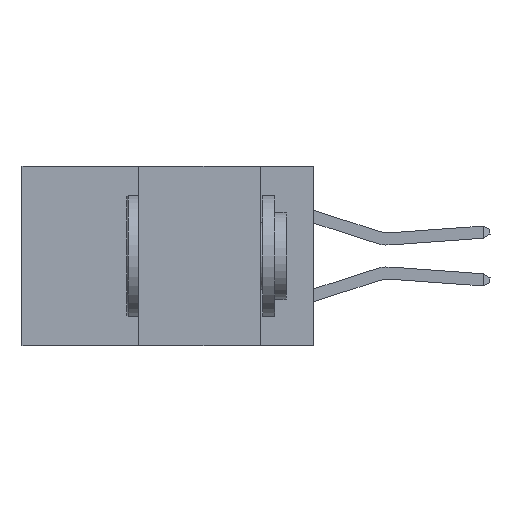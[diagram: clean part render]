
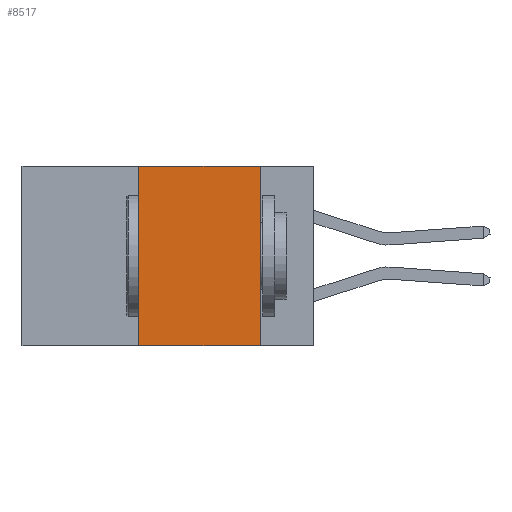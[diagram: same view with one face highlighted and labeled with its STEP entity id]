
A CAD part, left-side view. The second image highlights one B-rep face of the part: STEP entity #8517.
In plain terms, the highlighted planar face has unit normal (-1, 0, 0).
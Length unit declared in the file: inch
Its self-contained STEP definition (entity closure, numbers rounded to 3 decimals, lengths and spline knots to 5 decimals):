
#255 = AXIS2_PLACEMENT_3D ( 'NONE', #11285, #4114, #12508 ) ;
#1003 = LINE ( 'NONE', #3330, #7135 ) ;
#1275 = EDGE_CURVE ( 'NONE', #9500, #12603, #1003, .T. ) ;
#1798 = ORIENTED_EDGE ( 'NONE', *, *, #6247, .T. ) ;
#2509 = DIRECTION ( 'NONE',  ( 0., 0., -1. ) ) ;
#2677 = CARTESIAN_POINT ( 'NONE',  ( 0., 0.11, 0. ) ) ;
#2842 = VECTOR ( 'NONE', #13228, 39.37008 ) ;
#2998 = EDGE_CURVE ( 'NONE', #8325, #4891, #12520, .T. ) ;
#3330 = CARTESIAN_POINT ( 'NONE',  ( 0., 0.36, 0. ) ) ;
#3444 = FACE_OUTER_BOUND ( 'NONE', #7286, .T. ) ;
#3477 = DIRECTION ( 'NONE',  ( 0., 0., 1. ) ) ;
#3578 = CARTESIAN_POINT ( 'NONE',  ( 0., 0.36, -0.37 ) ) ;
#3944 = ORIENTED_EDGE ( 'NONE', *, *, #2998, .F. ) ;
#4114 = DIRECTION ( 'NONE',  ( 1., 0., 0. ) ) ;
#4818 = EDGE_CURVE ( 'NONE', #12603, #8325, #15138, .T. ) ;
#4891 = VERTEX_POINT ( 'NONE', #10911 ) ;
#6031 = LINE ( 'NONE', #7050, #9202 ) ;
#6247 = EDGE_CURVE ( 'NONE', #9500, #4891, #6031, .T. ) ;
#7050 = CARTESIAN_POINT ( 'NONE',  ( 0., 0.6, -0.37 ) ) ;
#7105 = ORIENTED_EDGE ( 'NONE', *, *, #4818, .F. ) ;
#7124 = DIRECTION ( 'NONE',  ( 0., -1., 0. ) ) ;
#7135 = VECTOR ( 'NONE', #3477, 39.37008 ) ;
#7286 = EDGE_LOOP ( 'NONE', ( #3944, #7105, #11058, #1798 ) ) ;
#7630 = PLANE ( 'NONE',  #255 ) ;
#8325 = VERTEX_POINT ( 'NONE', #9747 ) ;
#8517 = ADVANCED_FACE ( 'NONE', ( #3444 ), #7630, .F. ) ;
#9202 = VECTOR ( 'NONE', #7124, 39.37008 ) ;
#9500 = VERTEX_POINT ( 'NONE', #3578 ) ;
#9747 = CARTESIAN_POINT ( 'NONE',  ( 0., 0.11, 0. ) ) ;
#10460 = CARTESIAN_POINT ( 'NONE',  ( 0., 0.36, 0. ) ) ;
#10911 = CARTESIAN_POINT ( 'NONE',  ( 0., 0.11, -0.37 ) ) ;
#11058 = ORIENTED_EDGE ( 'NONE', *, *, #1275, .F. ) ;
#11285 = CARTESIAN_POINT ( 'NONE',  ( 0., 0.6, 0. ) ) ;
#12508 = DIRECTION ( 'NONE',  ( 0., 0., -1. ) ) ;
#12520 = LINE ( 'NONE', #2677, #15186 ) ;
#12603 = VERTEX_POINT ( 'NONE', #10460 ) ;
#12628 = CARTESIAN_POINT ( 'NONE',  ( 0., 0.6, 0. ) ) ;
#13228 = DIRECTION ( 'NONE',  ( 0., -1., 0. ) ) ;
#15138 = LINE ( 'NONE', #12628, #2842 ) ;
#15186 = VECTOR ( 'NONE', #2509, 39.37008 ) ;
